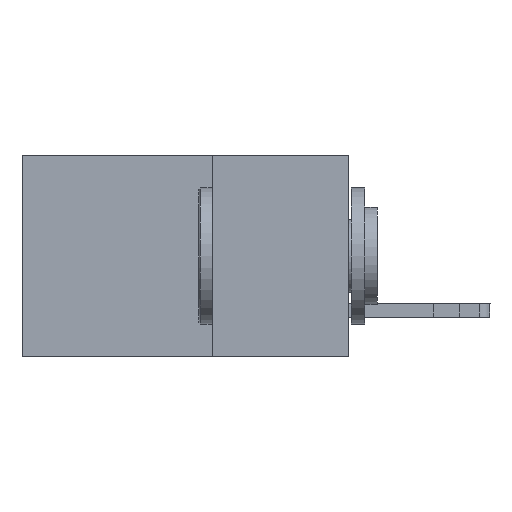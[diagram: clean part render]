
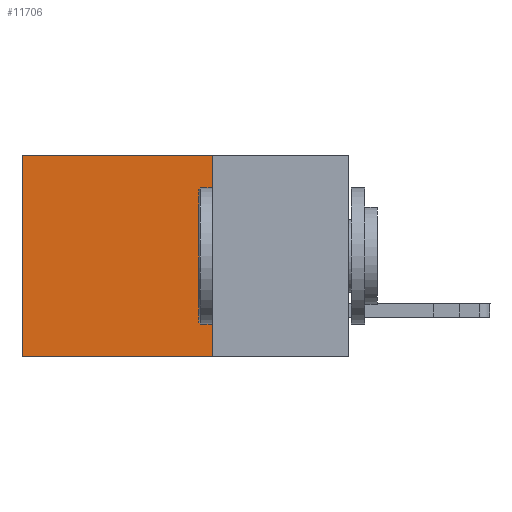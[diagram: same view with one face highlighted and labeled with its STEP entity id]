
A CAD part, left-side view. The second image highlights one B-rep face of the part: STEP entity #11706.
In plain terms, the highlighted planar face has unit normal (-1, 0, 0).
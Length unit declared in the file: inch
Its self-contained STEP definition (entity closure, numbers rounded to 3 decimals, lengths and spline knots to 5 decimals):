
#263 = DIRECTION ( 'NONE',  ( 0., 0., -1. ) ) ;
#974 = EDGE_CURVE ( 'NONE', #7039, #9316, #10564, .T. ) ;
#1082 = ORIENTED_EDGE ( 'NONE', *, *, #10823, .T. ) ;
#1538 = VERTEX_POINT ( 'NONE', #9809 ) ;
#3234 = CARTESIAN_POINT ( 'NONE',  ( 0.2615, 0.25, -0.37 ) ) ;
#3949 = CARTESIAN_POINT ( 'NONE',  ( 0.2615, 0.25, -0.37 ) ) ;
#5022 = LINE ( 'NONE', #3949, #10479 ) ;
#5196 = VERTEX_POINT ( 'NONE', #12575 ) ;
#5356 = FACE_OUTER_BOUND ( 'NONE', #12474, .T. ) ;
#6003 = VECTOR ( 'NONE', #7352, 39.37008 ) ;
#7039 = VERTEX_POINT ( 'NONE', #8318 ) ;
#7167 = DIRECTION ( 'NONE',  ( 0., 0., -1. ) ) ;
#7352 = DIRECTION ( 'NONE',  ( 0., 1., 0. ) ) ;
#7763 = VECTOR ( 'NONE', #10488, 39.37008 ) ;
#7862 = ORIENTED_EDGE ( 'NONE', *, *, #974, .F. ) ;
#8259 = PLANE ( 'NONE',  #10536 ) ;
#8318 = CARTESIAN_POINT ( 'NONE',  ( 0.2615, 0.25, -0.37 ) ) ;
#8536 = CARTESIAN_POINT ( 'NONE',  ( 0.2615, 0.6, -0.37 ) ) ;
#9130 = EDGE_CURVE ( 'NONE', #1538, #9316, #11564, .T. ) ;
#9272 = CARTESIAN_POINT ( 'NONE',  ( 0.2615, 0.25, -0.37 ) ) ;
#9316 = VERTEX_POINT ( 'NONE', #11486 ) ;
#9358 = LINE ( 'NONE', #11507, #6003 ) ;
#9473 = DIRECTION ( 'NONE',  ( 1., 0., 0. ) ) ;
#9620 = EDGE_CURVE ( 'NONE', #5196, #7039, #5022, .T. ) ;
#9809 = CARTESIAN_POINT ( 'NONE',  ( 0.2615, 0.6, 0. ) ) ;
#10479 = VECTOR ( 'NONE', #7167, 39.37008 ) ;
#10488 = DIRECTION ( 'NONE',  ( 0., 1., 0. ) ) ;
#10536 = AXIS2_PLACEMENT_3D ( 'NONE', #9272, #9473, #263 ) ;
#10564 = LINE ( 'NONE', #3234, #7763 ) ;
#10682 = ORIENTED_EDGE ( 'NONE', *, *, #9620, .F. ) ;
#10766 = DIRECTION ( 'NONE',  ( 0., 0., -1. ) ) ;
#10823 = EDGE_CURVE ( 'NONE', #5196, #1538, #9358, .T. ) ;
#10897 = VECTOR ( 'NONE', #10766, 39.37008 ) ;
#11486 = CARTESIAN_POINT ( 'NONE',  ( 0.2615, 0.6, -0.37 ) ) ;
#11507 = CARTESIAN_POINT ( 'NONE',  ( 0.2615, 0.25, 0. ) ) ;
#11522 = ORIENTED_EDGE ( 'NONE', *, *, #9130, .T. ) ;
#11564 = LINE ( 'NONE', #8536, #10897 ) ;
#11706 = ADVANCED_FACE ( 'NONE', ( #5356 ), #8259, .F. ) ;
#12474 = EDGE_LOOP ( 'NONE', ( #11522, #7862, #10682, #1082 ) ) ;
#12575 = CARTESIAN_POINT ( 'NONE',  ( 0.2615, 0.25, 0. ) ) ;
